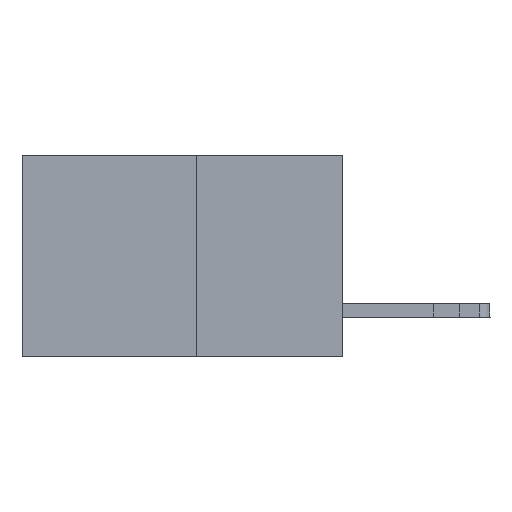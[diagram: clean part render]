
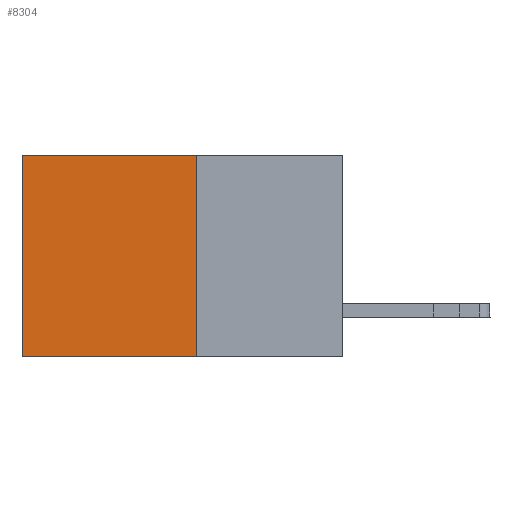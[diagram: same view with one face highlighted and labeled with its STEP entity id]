
A CAD part, left-side view. The second image highlights one B-rep face of the part: STEP entity #8304.
In plain terms, the highlighted planar face has unit normal (-1, 0, 0).
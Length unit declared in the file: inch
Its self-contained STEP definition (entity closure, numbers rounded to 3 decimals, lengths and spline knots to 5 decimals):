
#417 = VERTEX_POINT ( 'NONE', #7428 ) ;
#1332 = ORIENTED_EDGE ( 'NONE', *, *, #5029, .T. ) ;
#1611 = DIRECTION ( 'NONE',  ( 0., 1., 0. ) ) ;
#1720 = EDGE_CURVE ( 'NONE', #417, #14087, #15653, .T. ) ;
#1766 = CARTESIAN_POINT ( 'NONE',  ( 0.277, 0.59, 0. ) ) ;
#2171 = VECTOR ( 'NONE', #15506, 39.37008 ) ;
#2280 = CARTESIAN_POINT ( 'NONE',  ( 0.277, 0.27, 0. ) ) ;
#3039 = DIRECTION ( 'NONE',  ( 0., 0., -1. ) ) ;
#3324 = ORIENTED_EDGE ( 'NONE', *, *, #9090, .F. ) ;
#3356 = CARTESIAN_POINT ( 'NONE',  ( 0.277, 0.59, -0.37 ) ) ;
#3471 = VECTOR ( 'NONE', #7442, 39.37008 ) ;
#3910 = LINE ( 'NONE', #5285, #3471 ) ;
#3943 = ORIENTED_EDGE ( 'NONE', *, *, #1720, .T. ) ;
#4154 = CARTESIAN_POINT ( 'NONE',  ( 0.277, 0.27, -0.37 ) ) ;
#4207 = AXIS2_PLACEMENT_3D ( 'NONE', #4154, #6642, #3039 ) ;
#5029 = EDGE_CURVE ( 'NONE', #14087, #12391, #3910, .T. ) ;
#5285 = CARTESIAN_POINT ( 'NONE',  ( 0.277, 0.59, -0.37 ) ) ;
#6642 = DIRECTION ( 'NONE',  ( 1., 0., 0. ) ) ;
#7428 = CARTESIAN_POINT ( 'NONE',  ( 0.277, 0.27, 0. ) ) ;
#7442 = DIRECTION ( 'NONE',  ( 0., 0., -1. ) ) ;
#8304 = ADVANCED_FACE ( 'NONE', ( #10216 ), #15127, .F. ) ;
#9090 = EDGE_CURVE ( 'NONE', #417, #13032, #11879, .T. ) ;
#9352 = EDGE_CURVE ( 'NONE', #13032, #12391, #14917, .T. ) ;
#10216 = FACE_OUTER_BOUND ( 'NONE', #15007, .T. ) ;
#10620 = CARTESIAN_POINT ( 'NONE',  ( 0.277, 0.27, -0.37 ) ) ;
#11879 = LINE ( 'NONE', #15273, #2171 ) ;
#12146 = VECTOR ( 'NONE', #1611, 39.37008 ) ;
#12198 = DIRECTION ( 'NONE',  ( 0., 1., 0. ) ) ;
#12346 = CARTESIAN_POINT ( 'NONE',  ( 0.277, 0.27, -0.37 ) ) ;
#12391 = VERTEX_POINT ( 'NONE', #3356 ) ;
#12845 = ORIENTED_EDGE ( 'NONE', *, *, #9352, .F. ) ;
#13032 = VERTEX_POINT ( 'NONE', #10620 ) ;
#14087 = VERTEX_POINT ( 'NONE', #1766 ) ;
#14169 = VECTOR ( 'NONE', #12198, 39.37008 ) ;
#14917 = LINE ( 'NONE', #12346, #12146 ) ;
#15007 = EDGE_LOOP ( 'NONE', ( #1332, #12845, #3324, #3943 ) ) ;
#15127 = PLANE ( 'NONE',  #4207 ) ;
#15273 = CARTESIAN_POINT ( 'NONE',  ( 0.277, 0.27, -0.37 ) ) ;
#15506 = DIRECTION ( 'NONE',  ( 0., 0., -1. ) ) ;
#15653 = LINE ( 'NONE', #2280, #14169 ) ;
